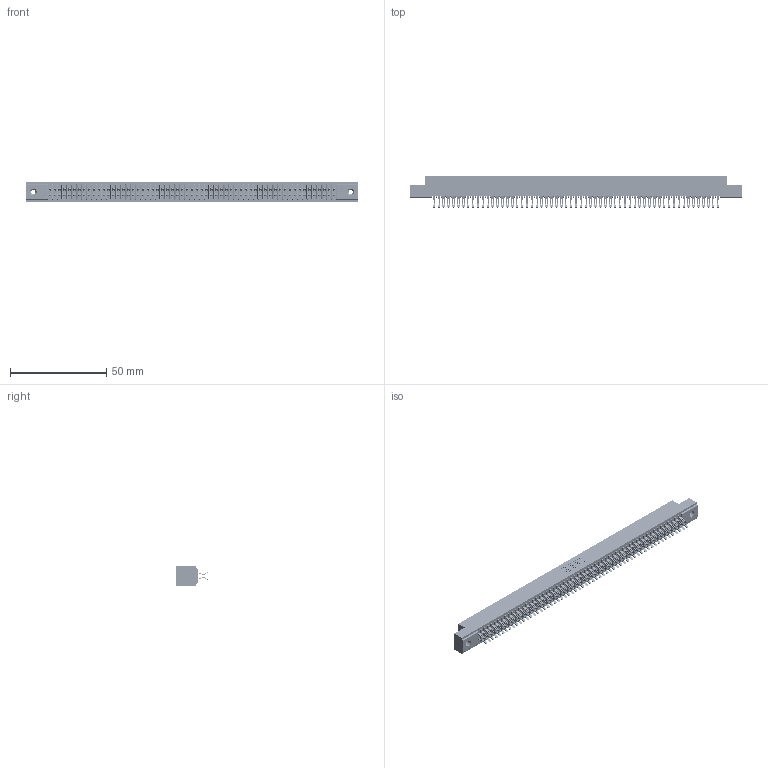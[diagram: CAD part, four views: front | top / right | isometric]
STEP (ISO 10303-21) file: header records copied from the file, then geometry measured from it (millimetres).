
FILE_DESCRIPTION (( 'STEP AP203' ), '1' );
FILE_NAME ('391-118-555-208.STEP', '2018-08-09T23:51:28', ( '' ), ( '' ), 'SwSTEP 2.0', 'SolidWorks 2016', '' );
FILE_SCHEMA (( 'CONFIG_CONTROL_DESIGN' ));
Products named in the file (4): 341-292-001_341-292-155; 345-250-001_345-250-003-102; 391-118-555-208; 341 Part_.156 (3.96) Dia Mounting Holes
Assembly tree (121 placements, depth 2):
  391-118-555-208
    341 Part_.156 (3.96) Dia Mounting Holes
    341-292-001_341-292-155  x118
    345-250-001_345-250-003-102  x2
Bounding box: 172.09 x 16.31 x 10.16 mm (x, y, z)
Volume: 12866.1 mm3; surface area: 24357.3 mm2
Topology: 121 solids, 121 shells, 9380 faces, 28005 edges, 18226 vertices
Faces by surface type: plane 5056, cylinder 4072, sphere 120, torus 120, cone 12
Entity records: 70793 total; most frequent: CARTESIAN_POINT 11766, ORIENTED_EDGE 11678, DIRECTION 11407, EDGE_CURVE 5839, LINE 4717, VECTOR 4717, VERTEX_POINT 3688, AXIS2_PLACEMENT_3D 3345
